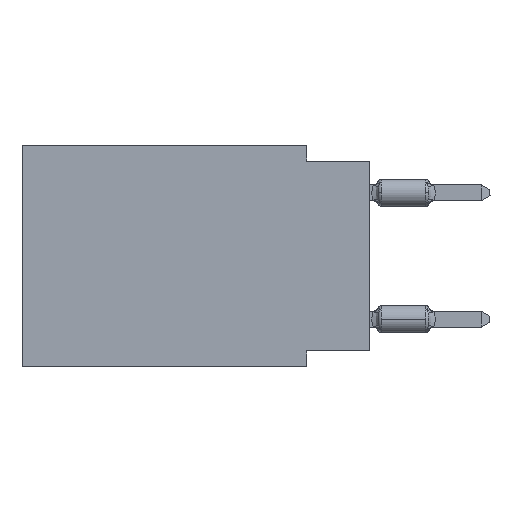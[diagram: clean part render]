
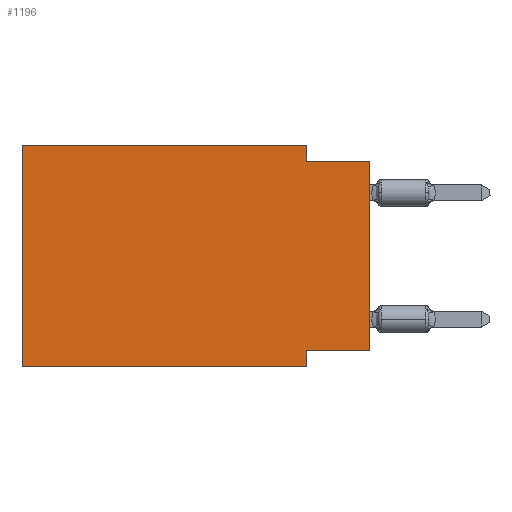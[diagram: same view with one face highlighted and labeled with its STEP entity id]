
A CAD part, left-side view. The second image highlights one B-rep face of the part: STEP entity #1196.
In plain terms, the highlighted planar face has unit normal (-1, 0, 0).
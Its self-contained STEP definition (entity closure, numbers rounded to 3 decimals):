
#403 = DIRECTION ( 'NONE',  ( 0., 0., -1. ) ) ;
#941 = ORIENTED_EDGE ( 'NONE', *, *, #27188, .F. ) ;
#1025 = ORIENTED_EDGE ( 'NONE', *, *, #18178, .F. ) ;
#1121 = FACE_OUTER_BOUND ( 'NONE', #43698, .T. ) ;
#1196 = ADVANCED_FACE ( 'NONE', ( #1121 ), #14920, .F. ) ;
#1779 = DIRECTION ( 'NONE',  ( 1., 0., 0. ) ) ;
#1889 = VECTOR ( 'NONE', #33360, 1000. ) ;
#1950 = LINE ( 'NONE', #32703, #14496 ) ;
#2234 = LINE ( 'NONE', #21203, #40290 ) ;
#3314 = CARTESIAN_POINT ( 'NONE',  ( 0., 0., -8.255 ) ) ;
#3438 = LINE ( 'NONE', #24690, #41368 ) ;
#5713 = ORIENTED_EDGE ( 'NONE', *, *, #22466, .F. ) ;
#7430 = VERTEX_POINT ( 'NONE', #36409 ) ;
#9538 = VERTEX_POINT ( 'NONE', #12582 ) ;
#10984 = VERTEX_POINT ( 'NONE', #44111 ) ;
#12459 = DIRECTION ( 'NONE',  ( 0., 0., 1. ) ) ;
#12582 = CARTESIAN_POINT ( 'NONE',  ( 0., 13.97, 0. ) ) ;
#14487 = VECTOR ( 'NONE', #42768, 1000. ) ;
#14496 = VECTOR ( 'NONE', #39062, 1000. ) ;
#14733 = CARTESIAN_POINT ( 'NONE',  ( 0., 13.97, -8.89 ) ) ;
#14920 = PLANE ( 'NONE',  #42685 ) ;
#15217 = VERTEX_POINT ( 'NONE', #25441 ) ;
#16075 = LINE ( 'NONE', #36416, #26761 ) ;
#17818 = VERTEX_POINT ( 'NONE', #36867 ) ;
#17962 = CARTESIAN_POINT ( 'NONE',  ( 0., 2.54, 0. ) ) ;
#18178 = EDGE_CURVE ( 'NONE', #31162, #9538, #29740, .T. ) ;
#19650 = ORIENTED_EDGE ( 'NONE', *, *, #33753, .F. ) ;
#21203 = CARTESIAN_POINT ( 'NONE',  ( 0., 2.54, -8.89 ) ) ;
#21696 = EDGE_CURVE ( 'NONE', #7430, #27858, #31067, .T. ) ;
#22466 = EDGE_CURVE ( 'NONE', #42825, #10984, #33470, .T. ) ;
#23372 = EDGE_CURVE ( 'NONE', #27858, #17818, #3438, .T. ) ;
#24040 = ORIENTED_EDGE ( 'NONE', *, *, #21696, .F. ) ;
#24690 = CARTESIAN_POINT ( 'NONE',  ( 0., 0., -0.635 ) ) ;
#24877 = LINE ( 'NONE', #14733, #14487 ) ;
#25441 = CARTESIAN_POINT ( 'NONE',  ( 0., 2.54, -8.89 ) ) ;
#26761 = VECTOR ( 'NONE', #12459, 1000. ) ;
#27188 = EDGE_CURVE ( 'NONE', #9538, #7430, #1950, .T. ) ;
#27858 = VERTEX_POINT ( 'NONE', #33089 ) ;
#29039 = VECTOR ( 'NONE', #31738, 1000. ) ;
#29740 = LINE ( 'NONE', #44228, #1889 ) ;
#30065 = CARTESIAN_POINT ( 'NONE',  ( 0., 0., -8.255 ) ) ;
#31067 = LINE ( 'NONE', #17962, #29039 ) ;
#31162 = VERTEX_POINT ( 'NONE', #43444 ) ;
#31738 = DIRECTION ( 'NONE',  ( 0., 0., -1. ) ) ;
#32703 = CARTESIAN_POINT ( 'NONE',  ( 0., 13.97, 0. ) ) ;
#32745 = CARTESIAN_POINT ( 'NONE',  ( 0., 13.97, 0. ) ) ;
#33089 = CARTESIAN_POINT ( 'NONE',  ( 0., 2.54, -0.635 ) ) ;
#33360 = DIRECTION ( 'NONE',  ( 0., 0., 1. ) ) ;
#33470 = LINE ( 'NONE', #30065, #40697 ) ;
#33753 = EDGE_CURVE ( 'NONE', #10984, #15217, #2234, .T. ) ;
#34639 = DIRECTION ( 'NONE',  ( 0., -1., 0. ) ) ;
#36409 = CARTESIAN_POINT ( 'NONE',  ( 0., 2.54, 0. ) ) ;
#36416 = CARTESIAN_POINT ( 'NONE',  ( 0., 0., 0. ) ) ;
#36439 = EDGE_CURVE ( 'NONE', #31162, #15217, #24877, .T. ) ;
#36867 = CARTESIAN_POINT ( 'NONE',  ( 0., 0., -0.635 ) ) ;
#39062 = DIRECTION ( 'NONE',  ( 0., -1., 0. ) ) ;
#40290 = VECTOR ( 'NONE', #403, 1000. ) ;
#40697 = VECTOR ( 'NONE', #43889, 1000. ) ;
#41368 = VECTOR ( 'NONE', #34639, 1000. ) ;
#42210 = ORIENTED_EDGE ( 'NONE', *, *, #43415, .T. ) ;
#42502 = DIRECTION ( 'NONE',  ( 0., 0., -1. ) ) ;
#42685 = AXIS2_PLACEMENT_3D ( 'NONE', #32745, #1779, #42502 ) ;
#42768 = DIRECTION ( 'NONE',  ( 0., -1., 0. ) ) ;
#42825 = VERTEX_POINT ( 'NONE', #3314 ) ;
#42942 = ORIENTED_EDGE ( 'NONE', *, *, #23372, .F. ) ;
#43415 = EDGE_CURVE ( 'NONE', #42825, #17818, #16075, .T. ) ;
#43444 = CARTESIAN_POINT ( 'NONE',  ( 0., 13.97, -8.89 ) ) ;
#43580 = ORIENTED_EDGE ( 'NONE', *, *, #36439, .T. ) ;
#43698 = EDGE_LOOP ( 'NONE', ( #42210, #42942, #24040, #941, #1025, #43580, #19650, #5713 ) ) ;
#43889 = DIRECTION ( 'NONE',  ( 0., 1., 0. ) ) ;
#44111 = CARTESIAN_POINT ( 'NONE',  ( 0., 2.54, -8.255 ) ) ;
#44228 = CARTESIAN_POINT ( 'NONE',  ( 0., 13.97, 0. ) ) ;
